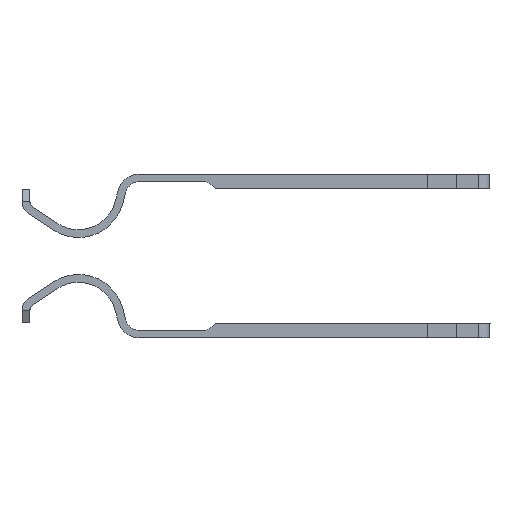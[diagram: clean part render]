
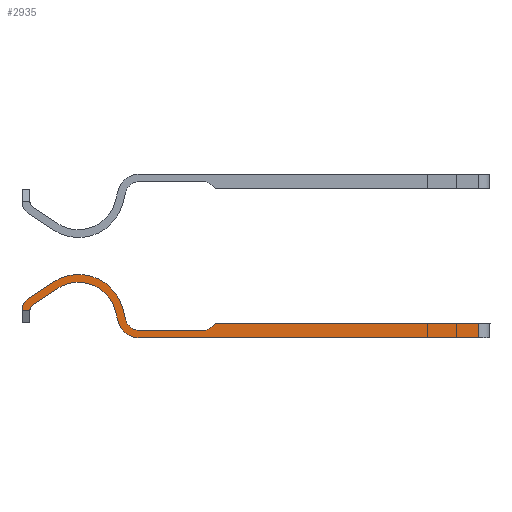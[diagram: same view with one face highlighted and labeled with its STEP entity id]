
A CAD part, left-side view. The second image highlights one B-rep face of the part: STEP entity #2935.
In plain terms, the highlighted face is planar.
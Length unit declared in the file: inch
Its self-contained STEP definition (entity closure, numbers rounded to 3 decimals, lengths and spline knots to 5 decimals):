
#189 = EDGE_CURVE ( 'NONE', #6344, #2159, #15226, .T. ) ;
#478 = DIRECTION ( 'NONE',  ( 0.836, 0.549, 0. ) ) ;
#497 = DIRECTION ( 'NONE',  ( 0.836, 0.549, 0. ) ) ;
#534 = VERTEX_POINT ( 'NONE', #12762 ) ;
#695 = CARTESIAN_POINT ( 'NONE',  ( 0.43721, 0.04723, 0.025 ) ) ;
#855 = DIRECTION ( 'NONE',  ( -0.707, -0.707, 0. ) ) ;
#936 = CIRCLE ( 'NONE', #8342, 0.0365 ) ;
#1173 = VECTOR ( 'NONE', #1293, 39.37008 ) ;
#1293 = DIRECTION ( 'NONE',  ( 0.268, -0.963, 0. ) ) ;
#1399 = CARTESIAN_POINT ( 'NONE',  ( 0.15971, 0.0575, 0.025 ) ) ;
#1449 = VECTOR ( 'NONE', #11576, 39.37008 ) ;
#1521 = VERTEX_POINT ( 'NONE', #2030 ) ;
#1629 = EDGE_CURVE ( 'NONE', #5482, #3964, #936, .T. ) ;
#1635 = DIRECTION ( 'NONE',  ( -1., 0., 0. ) ) ;
#1671 = CARTESIAN_POINT ( 'NONE',  ( 0.43721, 0.0255, 0.025 ) ) ;
#2030 = CARTESIAN_POINT ( 'NONE',  ( 0.89821, 0.0375, 0.025 ) ) ;
#2062 = EDGE_CURVE ( 'NONE', #534, #10459, #6102, .T. ) ;
#2159 = VERTEX_POINT ( 'NONE', #1671 ) ;
#2475 = DIRECTION ( 'NONE',  ( 1., 0., 0. ) ) ;
#2602 = ORIENTED_EDGE ( 'NONE', *, *, #10796, .F. ) ;
#2666 = VERTEX_POINT ( 'NONE', #9443 ) ;
#2701 = DIRECTION ( 'NONE',  ( -1., 0., 0. ) ) ;
#2904 = CARTESIAN_POINT ( 'NONE',  ( 0.228, 0.0425, 0.025 ) ) ;
#2935 = ADVANCED_FACE ( 'NONE', ( #15113 ), #7851, .F. ) ;
#3645 = ORIENTED_EDGE ( 'NONE', *, *, #10425, .F. ) ;
#3964 = VERTEX_POINT ( 'NONE', #15143 ) ;
#4083 = CARTESIAN_POINT ( 'NONE',  ( 0.33, 0.049, 0.025 ) ) ;
#4102 = VECTOR ( 'NONE', #6268, 39.37008 ) ;
#4216 = DIRECTION ( 'NONE',  ( -1., 0., 0. ) ) ;
#4297 = CARTESIAN_POINT ( 'NONE',  ( 0.14518, 0.07966, 0.025 ) ) ;
#4440 = VECTOR ( 'NONE', #6578, 39.37008 ) ;
#4555 = ORIENTED_EDGE ( 'NONE', *, *, #13029, .T. ) ;
#4577 = CARTESIAN_POINT ( 'NONE',  ( 0.33, 0.0255, 0.025 ) ) ;
#4795 = EDGE_CURVE ( 'NONE', #2666, #10238, #10304, .T. ) ;
#4848 = DIRECTION ( 'NONE',  ( 0., 0., -1. ) ) ;
#4929 = DIRECTION ( 'NONE',  ( -1., 0., 0. ) ) ;
#5271 = CARTESIAN_POINT ( 'NONE',  ( 0.89821, 0.0125, 0.025 ) ) ;
#5364 = DIRECTION ( 'NONE',  ( 1., 0., 0. ) ) ;
#5479 = CARTESIAN_POINT ( 'NONE',  ( 0.095, 0.025, 0.025 ) ) ;
#5482 = VERTEX_POINT ( 'NONE', #6517 ) ;
#5617 = AXIS2_PLACEMENT_3D ( 'NONE', #2904, #11306, #4216 ) ;
#5620 = CARTESIAN_POINT ( 'NONE',  ( 0.228, 0.0425, 0.025 ) ) ;
#5641 = VERTEX_POINT ( 'NONE', #13804 ) ;
#5816 = DIRECTION ( 'NONE',  ( 1., 0., 0. ) ) ;
#5990 = ORIENTED_EDGE ( 'NONE', *, *, #10333, .F. ) ;
#6054 = ORIENTED_EDGE ( 'NONE', *, *, #1629, .T. ) ;
#6074 = CARTESIAN_POINT ( 'NONE',  ( 0.45821, 0.0375, 0.025 ) ) ;
#6088 = LINE ( 'NONE', #13162, #11566 ) ;
#6102 = CIRCLE ( 'NONE', #14425, 0.0135 ) ;
#6126 = AXIS2_PLACEMENT_3D ( 'NONE', #5620, #13739, #6811 ) ;
#6195 = DIRECTION ( 'NONE',  ( 1., 0., 0. ) ) ;
#6268 = DIRECTION ( 'NONE',  ( 1., 0., 0. ) ) ;
#6344 = VERTEX_POINT ( 'NONE', #14608 ) ;
#6517 = CARTESIAN_POINT ( 'NONE',  ( 0.29484, 0.0392, 0.025 ) ) ;
#6543 = LINE ( 'NONE', #7999, #15369 ) ;
#6578 = DIRECTION ( 'NONE',  ( 0.268, -0.963, 0. ) ) ;
#6717 = AXIS2_PLACEMENT_3D ( 'NONE', #5479, #9001, #1635 ) ;
#6776 = ORIENTED_EDGE ( 'NONE', *, *, #13698, .T. ) ;
#6811 = DIRECTION ( 'NONE',  ( -1., 0., 0. ) ) ;
#7001 = VECTOR ( 'NONE', #4929, 39.37008 ) ;
#7039 = VERTEX_POINT ( 'NONE', #8718 ) ;
#7295 = EDGE_CURVE ( 'NONE', #10459, #9138, #14004, .T. ) ;
#7446 = DIRECTION ( 'NONE',  ( 0., 0., -1. ) ) ;
#7597 = CARTESIAN_POINT ( 'NONE',  ( 0.15231, 0.06879, 0.025 ) ) ;
#7758 = CARTESIAN_POINT ( 'NONE',  ( 0.28917, 0.05955, 0.025 ) ) ;
#7851 = PLANE ( 'NONE',  #6717 ) ;
#7931 = VERTEX_POINT ( 'NONE', #5271 ) ;
#7999 = CARTESIAN_POINT ( 'NONE',  ( 0.14518, 0.07966, 0.025 ) ) ;
#8086 = ORIENTED_EDGE ( 'NONE', *, *, #2062, .T. ) ;
#8257 = CARTESIAN_POINT ( 'NONE',  ( 0.45821, 0.0375, 0.025 ) ) ;
#8342 = AXIS2_PLACEMENT_3D ( 'NONE', #12509, #11426, #10900 ) ;
#8718 = CARTESIAN_POINT ( 'NONE',  ( 0.45821, 0.0375, 0.025 ) ) ;
#9001 = DIRECTION ( 'NONE',  ( 0., 0., -1. ) ) ;
#9005 = ORIENTED_EDGE ( 'NONE', *, *, #7295, .T. ) ;
#9041 = VERTEX_POINT ( 'NONE', #4297 ) ;
#9138 = VERTEX_POINT ( 'NONE', #11525 ) ;
#9156 = CIRCLE ( 'NONE', #6126, 0.0635 ) ;
#9235 = EDGE_CURVE ( 'NONE', #15401, #2159, #13419, .T. ) ;
#9443 = CARTESIAN_POINT ( 'NONE',  ( 0.18604, 0.10646, 0.025 ) ) ;
#9851 = EDGE_CURVE ( 'NONE', #13656, #5482, #13787, .T. ) ;
#9980 = DIRECTION ( 'NONE',  ( 0., 0., -1. ) ) ;
#10138 = EDGE_CURVE ( 'NONE', #7039, #6344, #14299, .T. ) ;
#10238 = VERTEX_POINT ( 'NONE', #11971 ) ;
#10304 = CIRCLE ( 'NONE', #5617, 0.0765 ) ;
#10333 = EDGE_CURVE ( 'NONE', #5641, #9041, #12162, .T. ) ;
#10425 = EDGE_CURVE ( 'NONE', #10238, #14886, #13620, .T. ) ;
#10459 = VERTEX_POINT ( 'NONE', #7597 ) ;
#10544 = VECTOR ( 'NONE', #855, 39.37008 ) ;
#10595 = ORIENTED_EDGE ( 'NONE', *, *, #10138, .T. ) ;
#10679 = CARTESIAN_POINT ( 'NONE',  ( 0.33, 0.0255, 0.025 ) ) ;
#10737 = CARTESIAN_POINT ( 'NONE',  ( 0.28917, 0.05955, 0.025 ) ) ;
#10796 = EDGE_CURVE ( 'NONE', #9041, #2666, #6543, .T. ) ;
#10845 = CIRCLE ( 'NONE', #15222, 0.0235 ) ;
#10900 = DIRECTION ( 'NONE',  ( 1., 0., 0. ) ) ;
#10943 = ORIENTED_EDGE ( 'NONE', *, *, #189, .T. ) ;
#10949 = VECTOR ( 'NONE', #497, 39.37008 ) ;
#11083 = VECTOR ( 'NONE', #5816, 39.37008 ) ;
#11153 = LINE ( 'NONE', #12742, #1449 ) ;
#11306 = DIRECTION ( 'NONE',  ( 0., 0., -1. ) ) ;
#11426 = DIRECTION ( 'NONE',  ( 0., 0., 1. ) ) ;
#11500 = ORIENTED_EDGE ( 'NONE', *, *, #15213, .F. ) ;
#11525 = CARTESIAN_POINT ( 'NONE',  ( 0.19317, 0.09559, 0.025 ) ) ;
#11566 = VECTOR ( 'NONE', #6195, 39.37008 ) ;
#11576 = DIRECTION ( 'NONE',  ( 0., -1., 0. ) ) ;
#11971 = CARTESIAN_POINT ( 'NONE',  ( 0.30169, 0.06304, 0.025 ) ) ;
#11986 = AXIS2_PLACEMENT_3D ( 'NONE', #14351, #7446, #15487 ) ;
#12078 = CARTESIAN_POINT ( 'NONE',  ( 0.33, 0.0125, 0.025 ) ) ;
#12162 = CIRCLE ( 'NONE', #11986, 0.0265 ) ;
#12202 = ORIENTED_EDGE ( 'NONE', *, *, #13119, .F. ) ;
#12216 = CARTESIAN_POINT ( 'NONE',  ( 0.30169, 0.06304, 0.025 ) ) ;
#12346 = DIRECTION ( 'NONE',  ( 0., 0., 1. ) ) ;
#12509 = CARTESIAN_POINT ( 'NONE',  ( 0.33, 0.049, 0.025 ) ) ;
#12742 = CARTESIAN_POINT ( 'NONE',  ( 0.89821, 0.37918, 0.025 ) ) ;
#12762 = CARTESIAN_POINT ( 'NONE',  ( 0.14622, 0.058, 0.025 ) ) ;
#13029 = EDGE_CURVE ( 'NONE', #5641, #534, #6088, .T. ) ;
#13119 = EDGE_CURVE ( 'NONE', #14886, #15401, #10845, .T. ) ;
#13151 = LINE ( 'NONE', #12078, #4102 ) ;
#13162 = CARTESIAN_POINT ( 'NONE',  ( 0.14621, 0.058, 0.025 ) ) ;
#13419 = LINE ( 'NONE', #4577, #11083 ) ;
#13532 = LINE ( 'NONE', #6074, #7001 ) ;
#13620 = LINE ( 'NONE', #12216, #1173 ) ;
#13656 = VERTEX_POINT ( 'NONE', #10737 ) ;
#13698 = EDGE_CURVE ( 'NONE', #1521, #7039, #13532, .T. ) ;
#13739 = DIRECTION ( 'NONE',  ( 0., 0., -1. ) ) ;
#13787 = LINE ( 'NONE', #7758, #4440 ) ;
#13804 = CARTESIAN_POINT ( 'NONE',  ( 0.13322, 0.058, 0.025 ) ) ;
#14004 = LINE ( 'NONE', #14892, #10949 ) ;
#14033 = ORIENTED_EDGE ( 'NONE', *, *, #14722, .T. ) ;
#14055 = ORIENTED_EDGE ( 'NONE', *, *, #15103, .T. ) ;
#14299 = LINE ( 'NONE', #8257, #10544 ) ;
#14351 = CARTESIAN_POINT ( 'NONE',  ( 0.15971, 0.0575, 0.025 ) ) ;
#14425 = AXIS2_PLACEMENT_3D ( 'NONE', #1399, #9980, #2701 ) ;
#14498 = ORIENTED_EDGE ( 'NONE', *, *, #4795, .F. ) ;
#14544 = CARTESIAN_POINT ( 'NONE',  ( 0.30736, 0.04269, 0.025 ) ) ;
#14573 = AXIS2_PLACEMENT_3D ( 'NONE', #695, #4848, #2475 ) ;
#14608 = CARTESIAN_POINT ( 'NONE',  ( 0.45258, 0.03186, 0.025 ) ) ;
#14681 = ORIENTED_EDGE ( 'NONE', *, *, #9235, .F. ) ;
#14722 = EDGE_CURVE ( 'NONE', #3964, #7931, #13151, .T. ) ;
#14857 = EDGE_LOOP ( 'NONE', ( #5990, #4555, #8086, #9005, #14055, #14924, #6054, #14033, #11500, #6776, #10595, #10943, #14681, #12202, #3645, #14498, #2602 ) ) ;
#14886 = VERTEX_POINT ( 'NONE', #14544 ) ;
#14892 = CARTESIAN_POINT ( 'NONE',  ( 0.15231, 0.06879, 0.025 ) ) ;
#14924 = ORIENTED_EDGE ( 'NONE', *, *, #9851, .T. ) ;
#15103 = EDGE_CURVE ( 'NONE', #9138, #13656, #9156, .T. ) ;
#15113 = FACE_OUTER_BOUND ( 'NONE', #14857, .T. ) ;
#15143 = CARTESIAN_POINT ( 'NONE',  ( 0.33, 0.0125, 0.025 ) ) ;
#15213 = EDGE_CURVE ( 'NONE', #1521, #7931, #11153, .T. ) ;
#15222 = AXIS2_PLACEMENT_3D ( 'NONE', #4083, #12346, #5364 ) ;
#15226 = CIRCLE ( 'NONE', #14573, 0.02173 ) ;
#15369 = VECTOR ( 'NONE', #478, 39.37008 ) ;
#15401 = VERTEX_POINT ( 'NONE', #10679 ) ;
#15487 = DIRECTION ( 'NONE',  ( -1., 0., 0. ) ) ;
